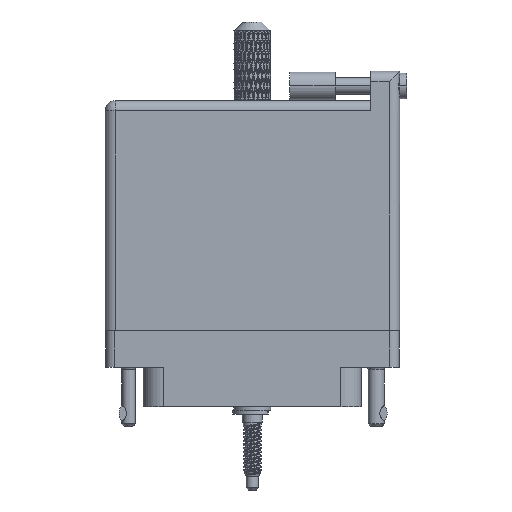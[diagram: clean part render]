
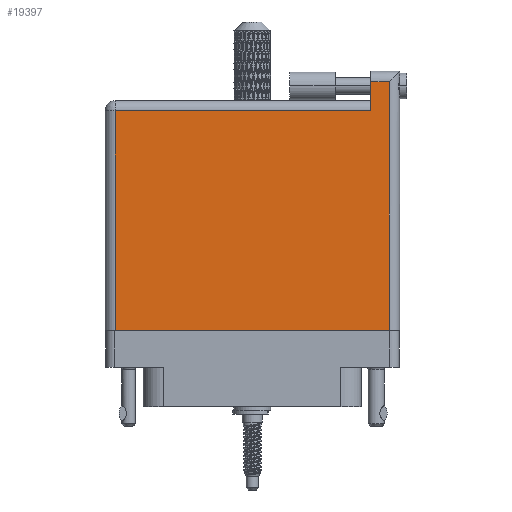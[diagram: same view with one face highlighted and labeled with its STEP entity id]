
A CAD part, front view. The second image highlights one B-rep face of the part: STEP entity #19397.
In plain terms, the highlighted face is planar.
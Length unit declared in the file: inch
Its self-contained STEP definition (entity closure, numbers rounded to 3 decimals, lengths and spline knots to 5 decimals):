
#1926 = EDGE_CURVE ( 'NONE', #97905, #86917, #112457, .T. ) ;
#5854 = CARTESIAN_POINT ( 'NONE',  ( -1.004, -0.1, 0.4495 ) ) ;
#6865 = VERTEX_POINT ( 'NONE', #98429 ) ;
#8444 = VECTOR ( 'NONE', #104600, 39.37008 ) ;
#10768 = LINE ( 'NONE', #105157, #17626 ) ;
#16980 = DIRECTION ( 'NONE',  ( 0., 0., -1. ) ) ;
#17626 = VECTOR ( 'NONE', #63272, 39.37008 ) ;
#18198 = LINE ( 'NONE', #5854, #8444 ) ;
#19397 = ADVANCED_FACE ( 'NONE', ( #19712 ), #78936, .F. ) ;
#19712 = FACE_OUTER_BOUND ( 'NONE', #42306, .T. ) ;
#21378 = CARTESIAN_POINT ( 'NONE',  ( 0.934, -0.1, 0.4495 ) ) ;
#25862 = CARTESIAN_POINT ( 'NONE',  ( -1.004, 1.466, 0.4495 ) ) ;
#28350 = LINE ( 'NONE', #85942, #81112 ) ;
#32865 = CARTESIAN_POINT ( 'NONE',  ( 0.807, 1.596, 0.4495 ) ) ;
#36966 = ORIENTED_EDGE ( 'NONE', *, *, #102390, .T. ) ;
#42306 = EDGE_LOOP ( 'NONE', ( #67689, #36966, #54581, #52141, #45405, #107537 ) ) ;
#43248 = EDGE_CURVE ( 'NONE', #111264, #6865, #10768, .T. ) ;
#45405 = ORIENTED_EDGE ( 'NONE', *, *, #77464, .T. ) ;
#51015 = DIRECTION ( 'NONE',  ( 0., 1., 0. ) ) ;
#52141 = ORIENTED_EDGE ( 'NONE', *, *, #53865, .T. ) ;
#52154 = CARTESIAN_POINT ( 'NONE',  ( 0.934, 1.596, 0.4495 ) ) ;
#53244 = DIRECTION ( 'NONE',  ( -1., 0., 0. ) ) ;
#53865 = EDGE_CURVE ( 'NONE', #86917, #93168, #93322, .T. ) ;
#54581 = ORIENTED_EDGE ( 'NONE', *, *, #1926, .T. ) ;
#56472 = EDGE_CURVE ( 'NONE', #6865, #60431, #18198, .T. ) ;
#57147 = CARTESIAN_POINT ( 'NONE',  ( -1.004, 1.596, 0.4495 ) ) ;
#57931 = DIRECTION ( 'NONE',  ( -1., 0., 0. ) ) ;
#58853 = VECTOR ( 'NONE', #92601, 39.37008 ) ;
#60431 = VERTEX_POINT ( 'NONE', #21378 ) ;
#63272 = DIRECTION ( 'NONE',  ( 0., -1., 0. ) ) ;
#64017 = VECTOR ( 'NONE', #57931, 39.37008 ) ;
#67689 = ORIENTED_EDGE ( 'NONE', *, *, #56472, .T. ) ;
#69791 = VECTOR ( 'NONE', #88329, 39.37008 ) ;
#77464 = EDGE_CURVE ( 'NONE', #93168, #111264, #106040, .T. ) ;
#78936 = PLANE ( 'NONE',  #79555 ) ;
#79555 = AXIS2_PLACEMENT_3D ( 'NONE', #25862, #16980, #53244 ) ;
#79833 = CARTESIAN_POINT ( 'NONE',  ( 0.807, 1.666, 0.4495 ) ) ;
#81112 = VECTOR ( 'NONE', #51015, 39.37008 ) ;
#85942 = CARTESIAN_POINT ( 'NONE',  ( 0.934, 1.666, 0.4495 ) ) ;
#86917 = VERTEX_POINT ( 'NONE', #32865 ) ;
#88329 = DIRECTION ( 'NONE',  ( 0., -1., 0. ) ) ;
#89918 = CARTESIAN_POINT ( 'NONE',  ( -0.934, 1.396, 0.4495 ) ) ;
#92601 = DIRECTION ( 'NONE',  ( -1., 0., 0. ) ) ;
#93168 = VERTEX_POINT ( 'NONE', #102748 ) ;
#93322 = LINE ( 'NONE', #79833, #69791 ) ;
#97905 = VERTEX_POINT ( 'NONE', #52154 ) ;
#98429 = CARTESIAN_POINT ( 'NONE',  ( -0.934, -0.1, 0.4495 ) ) ;
#100793 = CARTESIAN_POINT ( 'NONE',  ( -1.004, 1.396, 0.4495 ) ) ;
#102390 = EDGE_CURVE ( 'NONE', #60431, #97905, #28350, .T. ) ;
#102748 = CARTESIAN_POINT ( 'NONE',  ( 0.807, 1.396, 0.4495 ) ) ;
#104600 = DIRECTION ( 'NONE',  ( 1., 0., 0. ) ) ;
#105157 = CARTESIAN_POINT ( 'NONE',  ( -0.934, -0.1, 0.4495 ) ) ;
#106040 = LINE ( 'NONE', #100793, #58853 ) ;
#107537 = ORIENTED_EDGE ( 'NONE', *, *, #43248, .T. ) ;
#111264 = VERTEX_POINT ( 'NONE', #89918 ) ;
#112457 = LINE ( 'NONE', #57147, #64017 ) ;
